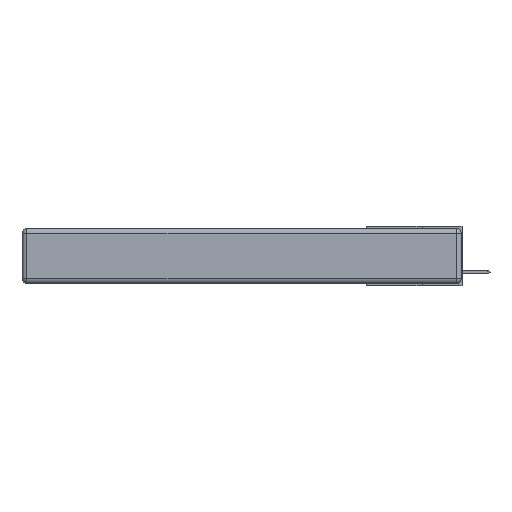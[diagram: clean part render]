
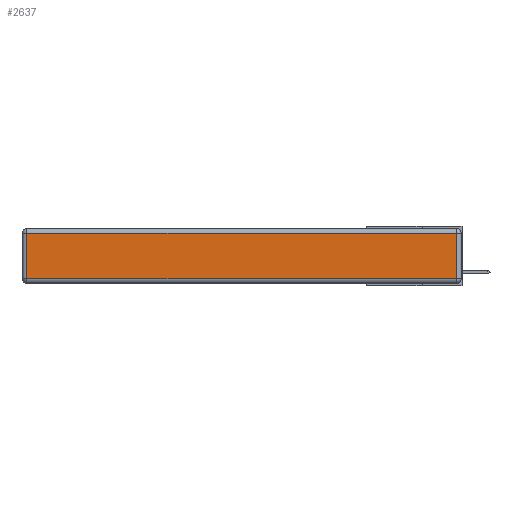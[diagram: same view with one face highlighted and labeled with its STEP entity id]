
A CAD part, left-side view. The second image highlights one B-rep face of the part: STEP entity #2637.
In plain terms, the highlighted planar face has unit normal (-1, 0, 0).
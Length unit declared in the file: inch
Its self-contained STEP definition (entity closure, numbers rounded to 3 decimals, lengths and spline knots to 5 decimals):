
#171 = CARTESIAN_POINT ( 'NONE',  ( 0., 0., -0.313 ) ) ;
#583 = EDGE_LOOP ( 'NONE', ( #2423, #10914, #13464, #1410 ) ) ;
#1379 = CARTESIAN_POINT ( 'NONE',  ( 0., 2.72, -0.313 ) ) ;
#1410 = ORIENTED_EDGE ( 'NONE', *, *, #14299, .T. ) ;
#1639 = VERTEX_POINT ( 'NONE', #6855 ) ;
#1887 = CARTESIAN_POINT ( 'NONE',  ( 0., 2.75, -0.03 ) ) ;
#2423 = ORIENTED_EDGE ( 'NONE', *, *, #5364, .T. ) ;
#2637 = ADVANCED_FACE ( 'NONE', ( #5910 ), #3174, .T. ) ;
#2933 = DIRECTION ( 'NONE',  ( 0., 0., 1. ) ) ;
#3174 = PLANE ( 'NONE',  #5179 ) ;
#3240 = LINE ( 'NONE', #12020, #7985 ) ;
#4864 = LINE ( 'NONE', #14581, #10335 ) ;
#5179 = AXIS2_PLACEMENT_3D ( 'NONE', #8948, #14781, #7626 ) ;
#5301 = VERTEX_POINT ( 'NONE', #14018 ) ;
#5364 = EDGE_CURVE ( 'NONE', #13651, #1639, #9676, .T. ) ;
#5910 = FACE_OUTER_BOUND ( 'NONE', #583, .T. ) ;
#6855 = CARTESIAN_POINT ( 'NONE',  ( 0., 0.03, -0.313 ) ) ;
#7626 = DIRECTION ( 'NONE',  ( 0., 0., 1. ) ) ;
#7985 = VECTOR ( 'NONE', #9846, 39.37008 ) ;
#8774 = VECTOR ( 'NONE', #11623, 39.37008 ) ;
#8948 = CARTESIAN_POINT ( 'NONE',  ( 0., 0., -0.343 ) ) ;
#9676 = LINE ( 'NONE', #171, #8774 ) ;
#9774 = CARTESIAN_POINT ( 'NONE',  ( 0., 2.72, -0.03 ) ) ;
#9842 = VECTOR ( 'NONE', #14422, 39.37008 ) ;
#9846 = DIRECTION ( 'NONE',  ( 0., 0., -1. ) ) ;
#10335 = VECTOR ( 'NONE', #2933, 39.37008 ) ;
#10751 = LINE ( 'NONE', #1887, #9842 ) ;
#10914 = ORIENTED_EDGE ( 'NONE', *, *, #14564, .T. ) ;
#11623 = DIRECTION ( 'NONE',  ( 0., -1., 0. ) ) ;
#12020 = CARTESIAN_POINT ( 'NONE',  ( 0., 2.72, -0.343 ) ) ;
#12191 = EDGE_CURVE ( 'NONE', #5301, #14864, #10751, .T. ) ;
#13464 = ORIENTED_EDGE ( 'NONE', *, *, #12191, .T. ) ;
#13651 = VERTEX_POINT ( 'NONE', #1379 ) ;
#14018 = CARTESIAN_POINT ( 'NONE',  ( 0., 0.03, -0.03 ) ) ;
#14299 = EDGE_CURVE ( 'NONE', #14864, #13651, #3240, .T. ) ;
#14422 = DIRECTION ( 'NONE',  ( 0., 1., 0. ) ) ;
#14564 = EDGE_CURVE ( 'NONE', #1639, #5301, #4864, .T. ) ;
#14581 = CARTESIAN_POINT ( 'NONE',  ( 0., 0.03, -0.343 ) ) ;
#14781 = DIRECTION ( 'NONE',  ( -1., 0., 0. ) ) ;
#14864 = VERTEX_POINT ( 'NONE', #9774 ) ;
